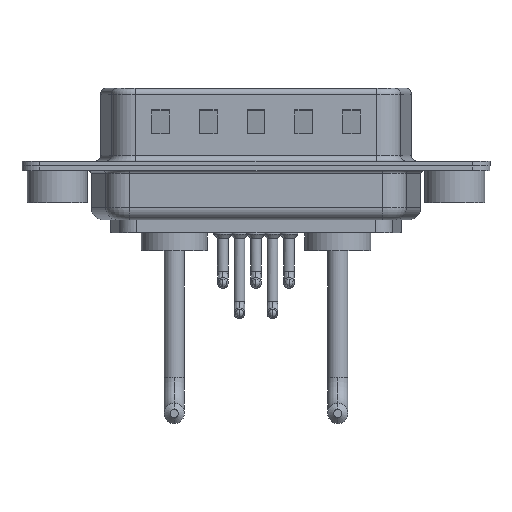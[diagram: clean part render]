
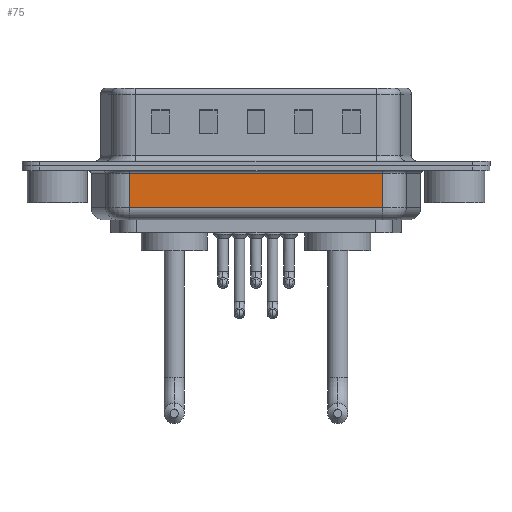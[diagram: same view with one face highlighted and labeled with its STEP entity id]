
A CAD part, front view. The second image highlights one B-rep face of the part: STEP entity #75.
In plain terms, the highlighted planar face has unit normal (0, -1, 0).
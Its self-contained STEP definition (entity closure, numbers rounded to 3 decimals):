
#71 = DIRECTION ( 'NONE',  ( 0., 0., 1. ) ) ;
#75 = ADVANCED_FACE ( 'NONE', ( #20746 ), #8150, .F. ) ;
#323 = EDGE_CURVE ( 'NONE', #16842, #11235, #3371, .T. ) ;
#638 = AXIS2_PLACEMENT_3D ( 'NONE', #6342, #6236, #71 ) ;
#2103 = CARTESIAN_POINT ( 'NONE',  ( 6.031, -5.35, -3.5 ) ) ;
#2136 = CARTESIAN_POINT ( 'NONE',  ( 6.031, -5.35, -0.65 ) ) ;
#2361 = VECTOR ( 'NONE', #3374, 1000. ) ;
#3058 = EDGE_CURVE ( 'NONE', #10220, #11235, #5112, .T. ) ;
#3371 = LINE ( 'NONE', #9848, #13516 ) ;
#3374 = DIRECTION ( 'NONE',  ( 1., 0., 0. ) ) ;
#3461 = CARTESIAN_POINT ( 'NONE',  ( 6.031, -5.35, -3.5 ) ) ;
#3483 = LINE ( 'NONE', #2103, #2361 ) ;
#5112 = LINE ( 'NONE', #2136, #8319 ) ;
#5868 = DIRECTION ( 'NONE',  ( 0., 0., 1. ) ) ;
#6114 = ORIENTED_EDGE ( 'NONE', *, *, #18748, .T. ) ;
#6130 = EDGE_CURVE ( 'NONE', #16842, #13614, #3483, .T. ) ;
#6236 = DIRECTION ( 'NONE',  ( 0., 1., 0. ) ) ;
#6342 = CARTESIAN_POINT ( 'NONE',  ( 6.031, -5.35, -4.5 ) ) ;
#8150 = PLANE ( 'NONE',  #638 ) ;
#8250 = EDGE_LOOP ( 'NONE', ( #19907, #14579, #6114, #15665 ) ) ;
#8319 = VECTOR ( 'NONE', #13143, 1000. ) ;
#9467 = LINE ( 'NONE', #20592, #16709 ) ;
#9848 = CARTESIAN_POINT ( 'NONE',  ( 6.031, -5.35, -4.5 ) ) ;
#10220 = VERTEX_POINT ( 'NONE', #19897 ) ;
#11235 = VERTEX_POINT ( 'NONE', #13341 ) ;
#13143 = DIRECTION ( 'NONE',  ( -1., 0., 0. ) ) ;
#13341 = CARTESIAN_POINT ( 'NONE',  ( 6.031, -5.35, -0.65 ) ) ;
#13516 = VECTOR ( 'NONE', #18217, 1000. ) ;
#13614 = VERTEX_POINT ( 'NONE', #18743 ) ;
#14579 = ORIENTED_EDGE ( 'NONE', *, *, #6130, .T. ) ;
#15665 = ORIENTED_EDGE ( 'NONE', *, *, #3058, .T. ) ;
#16709 = VECTOR ( 'NONE', #5868, 1000. ) ;
#16842 = VERTEX_POINT ( 'NONE', #3461 ) ;
#18217 = DIRECTION ( 'NONE',  ( 0., 0., 1. ) ) ;
#18743 = CARTESIAN_POINT ( 'NONE',  ( 27.269, -5.35, -3.5 ) ) ;
#18748 = EDGE_CURVE ( 'NONE', #13614, #10220, #9467, .T. ) ;
#19897 = CARTESIAN_POINT ( 'NONE',  ( 27.269, -5.35, -0.65 ) ) ;
#19907 = ORIENTED_EDGE ( 'NONE', *, *, #323, .F. ) ;
#20592 = CARTESIAN_POINT ( 'NONE',  ( 27.269, -5.35, -4.5 ) ) ;
#20746 = FACE_OUTER_BOUND ( 'NONE', #8250, .T. ) ;
